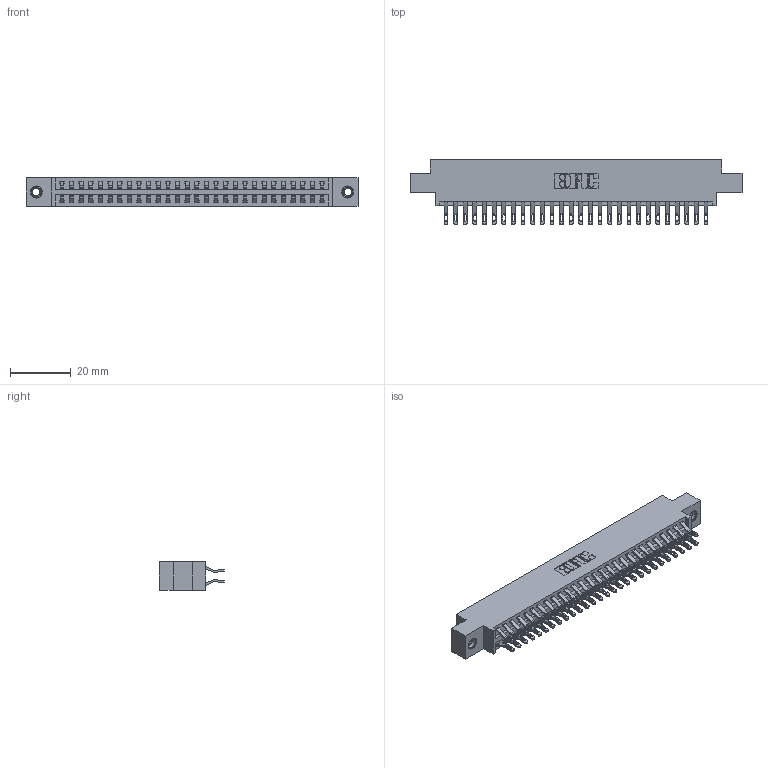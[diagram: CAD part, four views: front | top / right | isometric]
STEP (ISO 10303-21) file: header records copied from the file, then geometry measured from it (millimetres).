
FILE_DESCRIPTION (( 'STEP AP203' ), '1' );
FILE_NAME ('396-056-555-807.STEP', '2019-11-02T08:24:22', ( '' ), ( '' ), 'SwSTEP 2.0', 'SolidWorks 2016', '' );
FILE_SCHEMA (( 'CONFIG_CONTROL_DESIGN' ));
Length unit declared in the file: inch
Products named in the file (4): 346 Part_0.170 Offset - 0.156 Dia-TI; 345-292-001_555 Tail; 345-250-001_345-250-005-103; 396-056-555-807
Assembly tree (59 placements, depth 2):
  396-056-555-807
    346 Part_0.170 Offset - 0.156 Dia-TI
    345-292-001_555 Tail  x56
    345-250-001_345-250-005-103  x2
Bounding box: 109.47 x 21.46 x 9.4 mm (x, y, z)
Volume: 10560.6 mm3; surface area: 15088.6 mm2
Topology: 59 solids, 59 shells, 3434 faces, 10725 edges, 7142 vertices
Faces by surface type: plane 1960, cylinder 1458, cone 12, torus 4
Entity records: 21802 total; most frequent: CARTESIAN_POINT 3633, ORIENTED_EDGE 3530, DIRECTION 3247, EDGE_CURVE 1765, LINE 1481, VECTOR 1481, VERTEX_POINT 1172, AXIS2_PLACEMENT_3D 883
